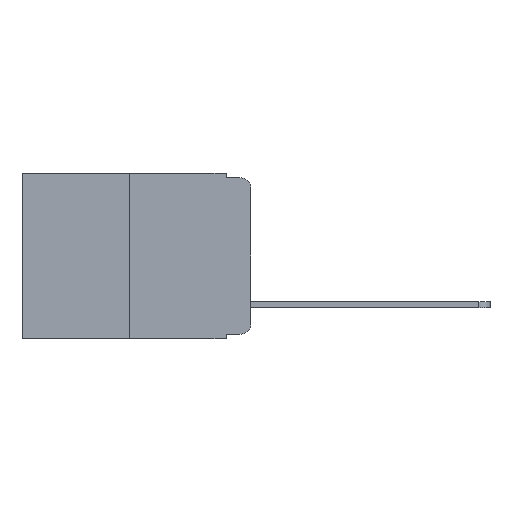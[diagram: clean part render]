
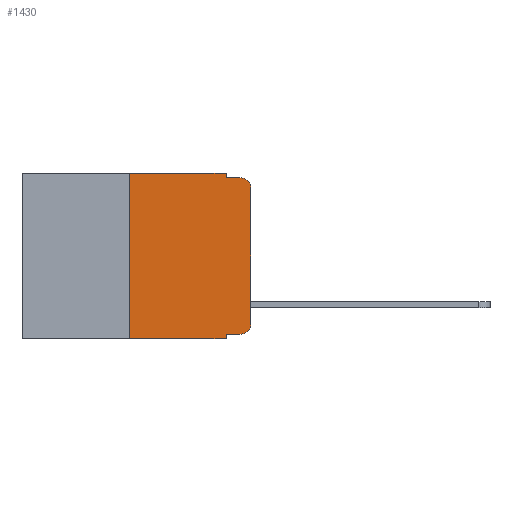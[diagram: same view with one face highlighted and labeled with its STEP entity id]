
A CAD part, left-side view. The second image highlights one B-rep face of the part: STEP entity #1430.
In plain terms, the highlighted planar face has unit normal (-1, 0, 0).
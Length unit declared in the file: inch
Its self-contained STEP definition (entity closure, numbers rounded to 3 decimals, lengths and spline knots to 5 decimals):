
#31 = CARTESIAN_POINT ( 'NONE',  ( 0., 0.051, -0.333 ) ) ;
#359 = CARTESIAN_POINT ( 'NONE',  ( 0., 0.02, -0.313 ) ) ;
#413 = VECTOR ( 'NONE', #10893, 39.37008 ) ;
#511 = VERTEX_POINT ( 'NONE', #13328 ) ;
#825 = VERTEX_POINT ( 'NONE', #3004 ) ;
#904 = CARTESIAN_POINT ( 'NONE',  ( 0., 0.473, -0.343 ) ) ;
#923 = CARTESIAN_POINT ( 'NONE',  ( 0., 0.051, 0. ) ) ;
#933 = LINE ( 'NONE', #3860, #9417 ) ;
#1205 = DIRECTION ( 'NONE',  ( -1., 0., 0. ) ) ;
#1312 = ORIENTED_EDGE ( 'NONE', *, *, #12453, .F. ) ;
#1420 = CARTESIAN_POINT ( 'NONE',  ( 0., 0.051, -0.333 ) ) ;
#1430 = ADVANCED_FACE ( 'NONE', ( #7730 ), #8778, .F. ) ;
#1553 = VERTEX_POINT ( 'NONE', #11160 ) ;
#1661 = DIRECTION ( 'NONE',  ( 0., 0., -1. ) ) ;
#1744 = CARTESIAN_POINT ( 'NONE',  ( 0., 0.051, -0.01 ) ) ;
#1912 = DIRECTION ( 'NONE',  ( 0., 0., 1. ) ) ;
#2082 = ORIENTED_EDGE ( 'NONE', *, *, #12515, .F. ) ;
#2248 = DIRECTION ( 'NONE',  ( 0., 0., -1. ) ) ;
#2289 = CARTESIAN_POINT ( 'NONE',  ( 0., 0.02, -0.333 ) ) ;
#2552 = ORIENTED_EDGE ( 'NONE', *, *, #11992, .F. ) ;
#3004 = CARTESIAN_POINT ( 'NONE',  ( 0., 0., -0.03 ) ) ;
#3368 = VERTEX_POINT ( 'NONE', #4829 ) ;
#3540 = VERTEX_POINT ( 'NONE', #12883 ) ;
#3572 = ORIENTED_EDGE ( 'NONE', *, *, #12313, .F. ) ;
#3815 = LINE ( 'NONE', #31, #413 ) ;
#3860 = CARTESIAN_POINT ( 'NONE',  ( 0., 0.473, 0. ) ) ;
#3886 = CARTESIAN_POINT ( 'NONE',  ( 0., 0.25, 0. ) ) ;
#3898 = CIRCLE ( 'NONE', #10413, 0.02 ) ;
#3941 = ORIENTED_EDGE ( 'NONE', *, *, #9228, .T. ) ;
#4126 = VERTEX_POINT ( 'NONE', #1420 ) ;
#4161 = ORIENTED_EDGE ( 'NONE', *, *, #8478, .F. ) ;
#4286 = ORIENTED_EDGE ( 'NONE', *, *, #12953, .T. ) ;
#4369 = LINE ( 'NONE', #904, #9192 ) ;
#4370 = AXIS2_PLACEMENT_3D ( 'NONE', #10552, #8762, #8311 ) ;
#4732 = ORIENTED_EDGE ( 'NONE', *, *, #8721, .T. ) ;
#4829 = CARTESIAN_POINT ( 'NONE',  ( 0., 0.051, -0.01 ) ) ;
#5211 = CIRCLE ( 'NONE', #10014, 0.02 ) ;
#5395 = CARTESIAN_POINT ( 'NONE',  ( 0., 0.051, 0. ) ) ;
#5467 = LINE ( 'NONE', #5395, #13311 ) ;
#5699 = ORIENTED_EDGE ( 'NONE', *, *, #8860, .T. ) ;
#5804 = VECTOR ( 'NONE', #10278, 39.37008 ) ;
#6354 = VECTOR ( 'NONE', #2248, 39.37008 ) ;
#6412 = DIRECTION ( 'NONE',  ( 0., 0., -1. ) ) ;
#6452 = VERTEX_POINT ( 'NONE', #11368 ) ;
#6559 = CARTESIAN_POINT ( 'NONE',  ( 0., 0.25, 0. ) ) ;
#6669 = EDGE_LOOP ( 'NONE', ( #10933, #4286, #1312, #2082, #2552, #3572, #3941, #4161, #4732, #5699 ) ) ;
#7730 = FACE_OUTER_BOUND ( 'NONE', #6669, .T. ) ;
#7817 = DIRECTION ( 'NONE',  ( 0., -1., 0. ) ) ;
#7819 = VERTEX_POINT ( 'NONE', #8401 ) ;
#8037 = CARTESIAN_POINT ( 'NONE',  ( 0., 0.02, -0.03 ) ) ;
#8076 = LINE ( 'NONE', #6559, #10817 ) ;
#8237 = VERTEX_POINT ( 'NONE', #3886 ) ;
#8311 = DIRECTION ( 'NONE',  ( 0., 0., -1. ) ) ;
#8352 = EDGE_CURVE ( 'NONE', #1553, #825, #13098, .T. ) ;
#8380 = DIRECTION ( 'NONE',  ( -1., 0., 0. ) ) ;
#8401 = CARTESIAN_POINT ( 'NONE',  ( 0., 0.051, -0.343 ) ) ;
#8478 = EDGE_CURVE ( 'NONE', #4126, #7819, #9318, .T. ) ;
#8550 = LINE ( 'NONE', #1744, #5804 ) ;
#8721 = EDGE_CURVE ( 'NONE', #4126, #9298, #3815, .T. ) ;
#8762 = DIRECTION ( 'NONE',  ( 1., 0., 0. ) ) ;
#8778 = PLANE ( 'NONE',  #4370 ) ;
#8860 = EDGE_CURVE ( 'NONE', #9298, #1553, #5211, .T. ) ;
#9015 = DIRECTION ( 'NONE',  ( 0., 0., -1. ) ) ;
#9067 = DIRECTION ( 'NONE',  ( 0., -1., 0. ) ) ;
#9192 = VECTOR ( 'NONE', #7817, 39.37008 ) ;
#9228 = EDGE_CURVE ( 'NONE', #511, #7819, #4369, .T. ) ;
#9298 = VERTEX_POINT ( 'NONE', #2289 ) ;
#9318 = LINE ( 'NONE', #923, #6354 ) ;
#9417 = VECTOR ( 'NONE', #9067, 39.37008 ) ;
#10014 = AXIS2_PLACEMENT_3D ( 'NONE', #359, #8380, #1661 ) ;
#10278 = DIRECTION ( 'NONE',  ( 0., -1., 0. ) ) ;
#10413 = AXIS2_PLACEMENT_3D ( 'NONE', #8037, #1205, #9015 ) ;
#10552 = CARTESIAN_POINT ( 'NONE',  ( 0., 0.473, 0. ) ) ;
#10742 = VECTOR ( 'NONE', #1912, 39.37008 ) ;
#10817 = VECTOR ( 'NONE', #13083, 39.37008 ) ;
#10893 = DIRECTION ( 'NONE',  ( 0., -1., 0. ) ) ;
#10933 = ORIENTED_EDGE ( 'NONE', *, *, #8352, .T. ) ;
#11160 = CARTESIAN_POINT ( 'NONE',  ( 0., 0., -0.313 ) ) ;
#11368 = CARTESIAN_POINT ( 'NONE',  ( 0., 0.02, -0.01 ) ) ;
#11992 = EDGE_CURVE ( 'NONE', #8237, #3540, #933, .T. ) ;
#12313 = EDGE_CURVE ( 'NONE', #511, #8237, #8076, .T. ) ;
#12453 = EDGE_CURVE ( 'NONE', #3368, #6452, #8550, .T. ) ;
#12515 = EDGE_CURVE ( 'NONE', #3540, #3368, #5467, .T. ) ;
#12883 = CARTESIAN_POINT ( 'NONE',  ( 0., 0.051, 0. ) ) ;
#12953 = EDGE_CURVE ( 'NONE', #825, #6452, #3898, .T. ) ;
#13030 = CARTESIAN_POINT ( 'NONE',  ( 0., 0., 0. ) ) ;
#13083 = DIRECTION ( 'NONE',  ( 0., 0., 1. ) ) ;
#13098 = LINE ( 'NONE', #13030, #10742 ) ;
#13311 = VECTOR ( 'NONE', #6412, 39.37008 ) ;
#13328 = CARTESIAN_POINT ( 'NONE',  ( 0., 0.25, -0.343 ) ) ;
